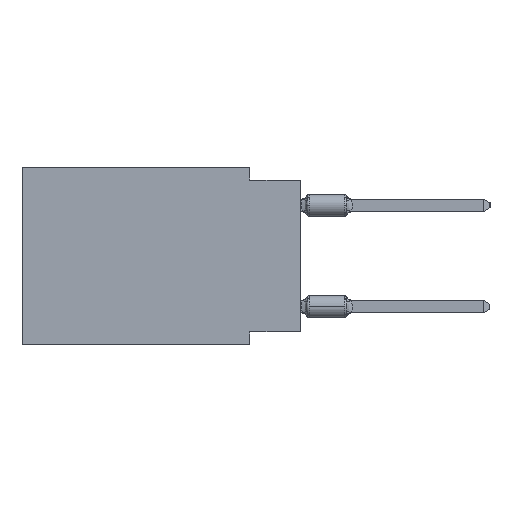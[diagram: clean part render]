
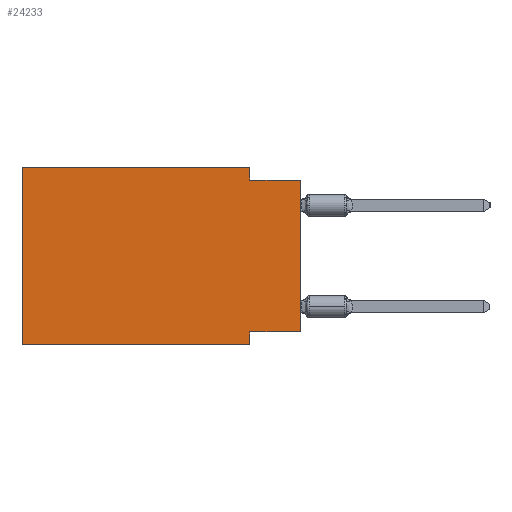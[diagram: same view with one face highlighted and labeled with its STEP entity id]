
A CAD part, left-side view. The second image highlights one B-rep face of the part: STEP entity #24233.
In plain terms, the highlighted planar face has unit normal (-1, 0, 0).
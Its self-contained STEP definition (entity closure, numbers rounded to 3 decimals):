
#530 = CARTESIAN_POINT ( 'NONE',  ( 0., 2.54, 0. ) ) ;
#1568 = ORIENTED_EDGE ( 'NONE', *, *, #34986, .F. ) ;
#1711 = ORIENTED_EDGE ( 'NONE', *, *, #17126, .F. ) ;
#1839 = VECTOR ( 'NONE', #22849, 1000. ) ;
#1847 = DIRECTION ( 'NONE',  ( 0., -1., 0. ) ) ;
#1907 = CARTESIAN_POINT ( 'NONE',  ( 0., 13.97, 0. ) ) ;
#2246 = EDGE_CURVE ( 'NONE', #10521, #22174, #32852, .T. ) ;
#2331 = CARTESIAN_POINT ( 'NONE',  ( 0., 13.97, 0. ) ) ;
#4982 = CARTESIAN_POINT ( 'NONE',  ( 0., 0., -8.255 ) ) ;
#5316 = FACE_OUTER_BOUND ( 'NONE', #10709, .T. ) ;
#6528 = LINE ( 'NONE', #19492, #15383 ) ;
#7550 = VERTEX_POINT ( 'NONE', #10127 ) ;
#8268 = VERTEX_POINT ( 'NONE', #18535 ) ;
#8879 = DIRECTION ( 'NONE',  ( 0., -1., 0. ) ) ;
#10127 = CARTESIAN_POINT ( 'NONE',  ( 0., 13.97, -8.89 ) ) ;
#10249 = EDGE_CURVE ( 'NONE', #22174, #36630, #21853, .T. ) ;
#10367 = EDGE_CURVE ( 'NONE', #7550, #41144, #38840, .T. ) ;
#10521 = VERTEX_POINT ( 'NONE', #21838 ) ;
#10709 = EDGE_LOOP ( 'NONE', ( #39113, #19935, #30309, #31974, #16880, #15937, #1568, #1711 ) ) ;
#10852 = VECTOR ( 'NONE', #19280, 1000. ) ;
#11551 = LINE ( 'NONE', #33896, #38614 ) ;
#12228 = CARTESIAN_POINT ( 'NONE',  ( 0., 13.97, -8.89 ) ) ;
#12918 = VECTOR ( 'NONE', #8879, 1000. ) ;
#13132 = CARTESIAN_POINT ( 'NONE',  ( 0., 2.54, -0.635 ) ) ;
#14486 = CARTESIAN_POINT ( 'NONE',  ( 0., 0., -0.635 ) ) ;
#14948 = DIRECTION ( 'NONE',  ( 0., 0., -1. ) ) ;
#15037 = CARTESIAN_POINT ( 'NONE',  ( 0., 0., -0.635 ) ) ;
#15383 = VECTOR ( 'NONE', #35857, 1000. ) ;
#15485 = CARTESIAN_POINT ( 'NONE',  ( 0., 0., 0. ) ) ;
#15937 = ORIENTED_EDGE ( 'NONE', *, *, #35783, .T. ) ;
#16274 = VECTOR ( 'NONE', #17991, 1000. ) ;
#16880 = ORIENTED_EDGE ( 'NONE', *, *, #10367, .F. ) ;
#17126 = EDGE_CURVE ( 'NONE', #30220, #39415, #6528, .T. ) ;
#17991 = DIRECTION ( 'NONE',  ( 0., -1., 0. ) ) ;
#18286 = DIRECTION ( 'NONE',  ( 1., 0., 0. ) ) ;
#18535 = CARTESIAN_POINT ( 'NONE',  ( 0., 2.54, -8.89 ) ) ;
#18821 = LINE ( 'NONE', #12228, #16274 ) ;
#19280 = DIRECTION ( 'NONE',  ( 0., 0., 1. ) ) ;
#19492 = CARTESIAN_POINT ( 'NONE',  ( 0., 0., -8.255 ) ) ;
#19935 = ORIENTED_EDGE ( 'NONE', *, *, #10249, .F. ) ;
#21838 = CARTESIAN_POINT ( 'NONE',  ( 0., 2.54, 0. ) ) ;
#21844 = LINE ( 'NONE', #31193, #27926 ) ;
#21853 = LINE ( 'NONE', #15037, #12918 ) ;
#22174 = VERTEX_POINT ( 'NONE', #13132 ) ;
#22849 = DIRECTION ( 'NONE',  ( 0., 0., -1. ) ) ;
#24233 = ADVANCED_FACE ( 'NONE', ( #5316 ), #28691, .F. ) ;
#27926 = VECTOR ( 'NONE', #1847, 1000. ) ;
#28114 = AXIS2_PLACEMENT_3D ( 'NONE', #1907, #18286, #41658 ) ;
#28532 = EDGE_CURVE ( 'NONE', #30220, #36630, #37808, .T. ) ;
#28691 = PLANE ( 'NONE',  #28114 ) ;
#30220 = VERTEX_POINT ( 'NONE', #4982 ) ;
#30309 = ORIENTED_EDGE ( 'NONE', *, *, #2246, .F. ) ;
#31193 = CARTESIAN_POINT ( 'NONE',  ( 0., 13.97, 0. ) ) ;
#31204 = VECTOR ( 'NONE', #35025, 1000. ) ;
#31974 = ORIENTED_EDGE ( 'NONE', *, *, #38608, .F. ) ;
#32852 = LINE ( 'NONE', #530, #1839 ) ;
#33896 = CARTESIAN_POINT ( 'NONE',  ( 0., 2.54, -8.89 ) ) ;
#34685 = CARTESIAN_POINT ( 'NONE',  ( 0., 2.54, -8.255 ) ) ;
#34986 = EDGE_CURVE ( 'NONE', #39415, #8268, #11551, .T. ) ;
#35025 = DIRECTION ( 'NONE',  ( 0., 0., 1. ) ) ;
#35223 = CARTESIAN_POINT ( 'NONE',  ( 0., 13.97, 0. ) ) ;
#35783 = EDGE_CURVE ( 'NONE', #7550, #8268, #18821, .T. ) ;
#35857 = DIRECTION ( 'NONE',  ( 0., 1., 0. ) ) ;
#36630 = VERTEX_POINT ( 'NONE', #14486 ) ;
#37808 = LINE ( 'NONE', #15485, #31204 ) ;
#38608 = EDGE_CURVE ( 'NONE', #41144, #10521, #21844, .T. ) ;
#38614 = VECTOR ( 'NONE', #14948, 1000. ) ;
#38840 = LINE ( 'NONE', #35223, #10852 ) ;
#39113 = ORIENTED_EDGE ( 'NONE', *, *, #28532, .T. ) ;
#39415 = VERTEX_POINT ( 'NONE', #34685 ) ;
#41144 = VERTEX_POINT ( 'NONE', #2331 ) ;
#41658 = DIRECTION ( 'NONE',  ( 0., 0., -1. ) ) ;
